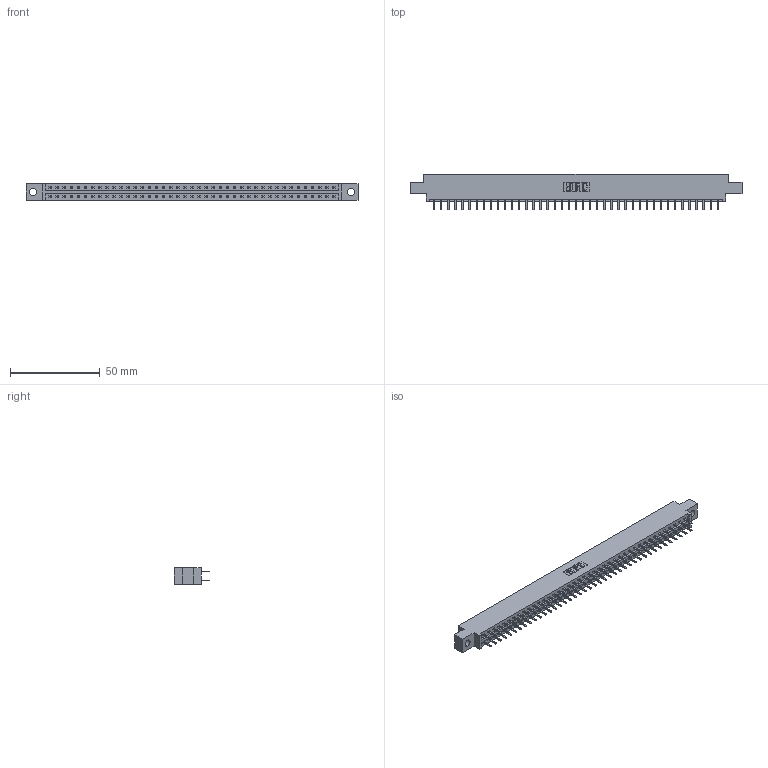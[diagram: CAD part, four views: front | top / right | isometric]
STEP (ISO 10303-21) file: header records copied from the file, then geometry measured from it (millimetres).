
FILE_DESCRIPTION (( 'STEP AP203' ), '1' );
FILE_NAME ('337-082-520-804.STEP', '2018-08-12T19:34:17', ( '' ), ( '' ), 'SwSTEP 2.0', 'SolidWorks 2016', '' );
FILE_SCHEMA (( 'CONFIG_CONTROL_DESIGN' ));
Length unit declared in the file: inch
Products named in the file (3): 345-292-001_345-293-120; 337-082-520-804; 337 Part_0.170 Offset - 0.156 Dia-TH
Assembly tree (83 placements, depth 2):
  337-082-520-804
    337 Part_0.170 Offset - 0.156 Dia-TH
    345-292-001_345-293-120  x82
Bounding box: 185.47 x 20.02 x 9.4 mm (x, y, z)
Volume: 19291.7 mm3; surface area: 21602 mm2
Topology: 83 solids, 83 shells, 4874 faces, 14181 edges, 9234 vertices
Faces by surface type: plane 3354, cylinder 1520
Entity records: 32167 total; most frequent: CARTESIAN_POINT 5434, ORIENTED_EDGE 5358, DIRECTION 4611, EDGE_CURVE 2679, VECTOR 2547, LINE 2547, VERTEX_POINT 1782, AXIS2_PLACEMENT_3D 1032
